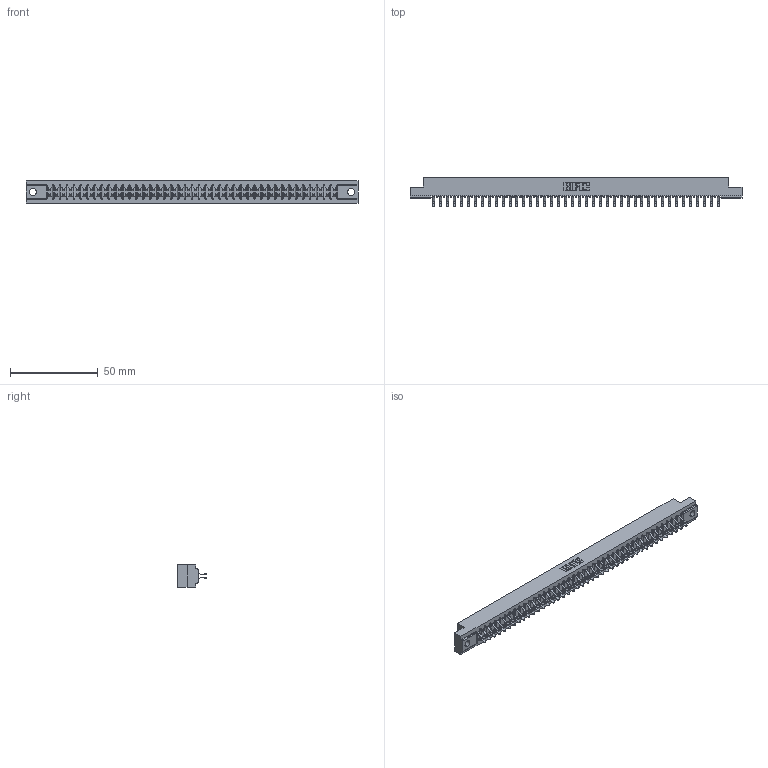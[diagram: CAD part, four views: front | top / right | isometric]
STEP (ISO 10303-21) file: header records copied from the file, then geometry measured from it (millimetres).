
FILE_DESCRIPTION (( 'STEP AP203' ), '1' );
FILE_NAME ('807-084-556-204.STEP', '2021-07-20T19:01:46', ( '' ), ( '' ), 'SwSTEP 2.0', 'SolidWorks 2020', '' );
FILE_SCHEMA (( 'CONFIG_CONTROL_DESIGN' ));
Length unit declared in the file: inch
Products named in the file (3): 807-084-556-204; 807 Part_.156 Dia Mounting Holes; 307-290-001_556
Assembly tree (85 placements, depth 2):
  807-084-556-204
    807 Part_.156 Dia Mounting Holes
    307-290-001_556  x84
Bounding box: 189.43 x 16.97 x 12.7 mm (x, y, z)
Volume: 20022.8 mm3; surface area: 24111.2 mm2
Topology: 85 solids, 85 shells, 4375 faces, 12287 edges, 7962 vertices
Faces by surface type: plane 2856, cylinder 1433, sphere 86
Entity records: 37872 total; most frequent: CARTESIAN_POINT 6200, ORIENTED_EDGE 6142, DIRECTION 6065, EDGE_CURVE 3071, VECTOR 2363, LINE 2363, VERTEX_POINT 1986, AXIS2_PLACEMENT_3D 1851
